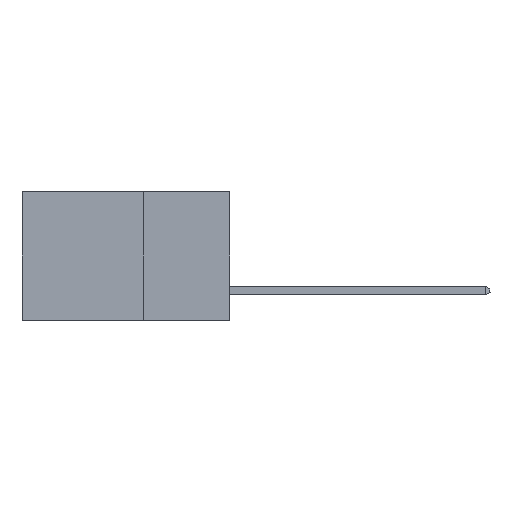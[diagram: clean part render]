
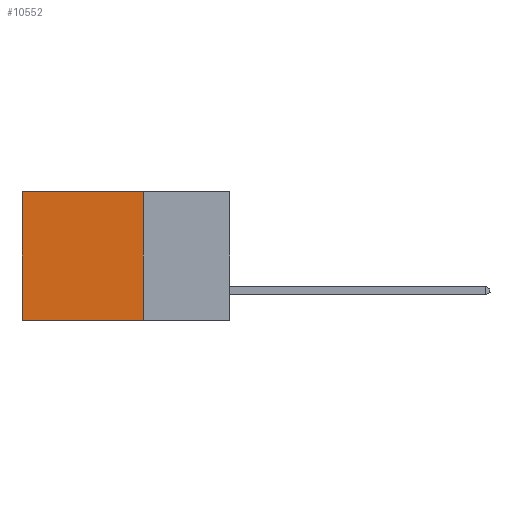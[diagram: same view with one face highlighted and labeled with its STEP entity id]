
A CAD part, left-side view. The second image highlights one B-rep face of the part: STEP entity #10552.
In plain terms, the highlighted planar face has unit normal (-1, 0, 0).
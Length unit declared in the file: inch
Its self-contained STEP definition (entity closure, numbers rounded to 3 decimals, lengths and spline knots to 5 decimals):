
#7 = DIRECTION ( 'NONE',  ( 1., 0., 0. ) ) ;
#54 = DIRECTION ( 'NONE',  ( 0., 0., -1. ) ) ;
#333 = LINE ( 'NONE', #2434, #717 ) ;
#509 = VERTEX_POINT ( 'NONE', #16863 ) ;
#526 = CARTESIAN_POINT ( 'NONE',  ( 0.298, 0.6, 0. ) ) ;
#686 = ORIENTED_EDGE ( 'NONE', *, *, #1022, .F. ) ;
#717 = VECTOR ( 'NONE', #3506, 39.37008 ) ;
#1014 = ORIENTED_EDGE ( 'NONE', *, *, #1239, .F. ) ;
#1022 = EDGE_CURVE ( 'NONE', #509, #14518, #333, .T. ) ;
#1239 = EDGE_CURVE ( 'NONE', #14518, #1501, #7350, .T. ) ;
#1501 = VERTEX_POINT ( 'NONE', #9319 ) ;
#2434 = CARTESIAN_POINT ( 'NONE',  ( 0.298, 0.25, 0. ) ) ;
#3506 = DIRECTION ( 'NONE',  ( 0., 0., -1. ) ) ;
#3644 = EDGE_LOOP ( 'NONE', ( #11333, #1014, #686, #4111 ) ) ;
#4111 = ORIENTED_EDGE ( 'NONE', *, *, #11913, .T. ) ;
#4129 = CARTESIAN_POINT ( 'NONE',  ( 0.298, 0.6, 0. ) ) ;
#4526 = FACE_OUTER_BOUND ( 'NONE', #3644, .T. ) ;
#5152 = VERTEX_POINT ( 'NONE', #4129 ) ;
#5699 = VECTOR ( 'NONE', #7114, 39.37008 ) ;
#5884 = CARTESIAN_POINT ( 'NONE',  ( 0.298, 0.25, -0.37 ) ) ;
#5969 = CARTESIAN_POINT ( 'NONE',  ( 0.298, 0.25, 0. ) ) ;
#6660 = CARTESIAN_POINT ( 'NONE',  ( 0.298, 0.25, 0. ) ) ;
#7114 = DIRECTION ( 'NONE',  ( 0., 1., 0. ) ) ;
#7203 = EDGE_CURVE ( 'NONE', #5152, #1501, #11031, .T. ) ;
#7350 = LINE ( 'NONE', #5884, #5699 ) ;
#9251 = CARTESIAN_POINT ( 'NONE',  ( 0.298, 0.25, -0.37 ) ) ;
#9319 = CARTESIAN_POINT ( 'NONE',  ( 0.298, 0.6, -0.37 ) ) ;
#10552 = ADVANCED_FACE ( 'NONE', ( #4526 ), #15914, .F. ) ;
#11031 = LINE ( 'NONE', #526, #11435 ) ;
#11333 = ORIENTED_EDGE ( 'NONE', *, *, #7203, .T. ) ;
#11435 = VECTOR ( 'NONE', #12362, 39.37008 ) ;
#11913 = EDGE_CURVE ( 'NONE', #509, #5152, #12570, .T. ) ;
#12362 = DIRECTION ( 'NONE',  ( 0., 0., -1. ) ) ;
#12480 = DIRECTION ( 'NONE',  ( 0., 1., 0. ) ) ;
#12570 = LINE ( 'NONE', #5969, #13570 ) ;
#13570 = VECTOR ( 'NONE', #12480, 39.37008 ) ;
#14518 = VERTEX_POINT ( 'NONE', #9251 ) ;
#15914 = PLANE ( 'NONE',  #16021 ) ;
#16021 = AXIS2_PLACEMENT_3D ( 'NONE', #6660, #7, #54 ) ;
#16863 = CARTESIAN_POINT ( 'NONE',  ( 0.298, 0.25, 0. ) ) ;
